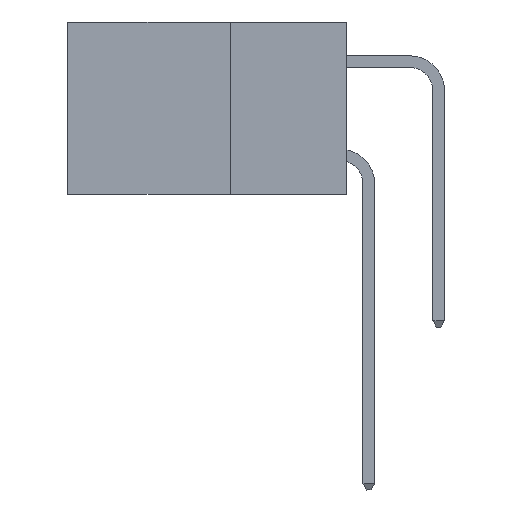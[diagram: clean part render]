
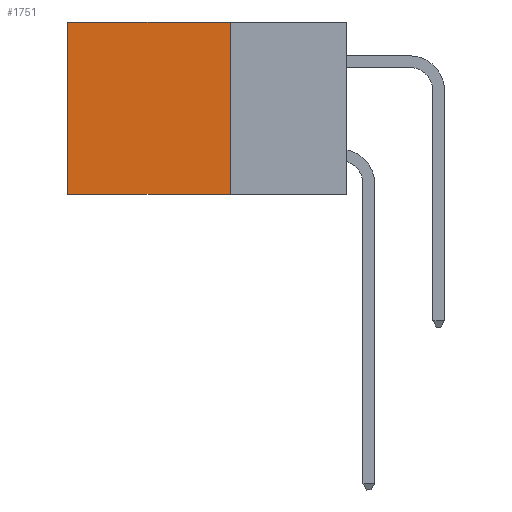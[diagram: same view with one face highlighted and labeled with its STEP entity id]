
A CAD part, left-side view. The second image highlights one B-rep face of the part: STEP entity #1751.
In plain terms, the highlighted planar face has unit normal (-1, 0, 0).
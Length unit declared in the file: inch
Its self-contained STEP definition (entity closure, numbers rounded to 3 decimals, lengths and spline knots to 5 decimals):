
#8 = DIRECTION ( 'NONE',  ( 0., 1., 0. ) ) ;
#408 = VERTEX_POINT ( 'NONE', #25837 ) ;
#820 = CARTESIAN_POINT ( 'NONE',  ( 0.2875, 0.25, -0.37 ) ) ;
#846 = VERTEX_POINT ( 'NONE', #19002 ) ;
#880 = FACE_OUTER_BOUND ( 'NONE', #23633, .T. ) ;
#1751 = ADVANCED_FACE ( 'NONE', ( #880 ), #26818, .F. ) ;
#1771 = VERTEX_POINT ( 'NONE', #12324 ) ;
#3113 = DIRECTION ( 'NONE',  ( 0., 0., -1. ) ) ;
#4030 = CARTESIAN_POINT ( 'NONE',  ( 0.2875, 0.25, 0. ) ) ;
#4594 = EDGE_CURVE ( 'NONE', #1771, #5830, #13624, .T. ) ;
#5017 = LINE ( 'NONE', #11598, #8546 ) ;
#5216 = VECTOR ( 'NONE', #19657, 39.37008 ) ;
#5830 = VERTEX_POINT ( 'NONE', #26468 ) ;
#8034 = CARTESIAN_POINT ( 'NONE',  ( 0.2875, 0.25, 0. ) ) ;
#8546 = VECTOR ( 'NONE', #11878, 39.37008 ) ;
#9437 = ORIENTED_EDGE ( 'NONE', *, *, #17806, .F. ) ;
#10472 = EDGE_CURVE ( 'NONE', #5830, #846, #19423, .T. ) ;
#11326 = CARTESIAN_POINT ( 'NONE',  ( 0.2875, 0.6, 0. ) ) ;
#11598 = CARTESIAN_POINT ( 'NONE',  ( 0.2875, 0.25, 0. ) ) ;
#11878 = DIRECTION ( 'NONE',  ( 0., 0., -1. ) ) ;
#12324 = CARTESIAN_POINT ( 'NONE',  ( 0.2875, 0.25, 0. ) ) ;
#13624 = LINE ( 'NONE', #8034, #25038 ) ;
#14179 = DIRECTION ( 'NONE',  ( 1., 0., 0. ) ) ;
#15277 = ORIENTED_EDGE ( 'NONE', *, *, #10472, .T. ) ;
#17806 = EDGE_CURVE ( 'NONE', #408, #846, #18508, .T. ) ;
#18508 = LINE ( 'NONE', #820, #5216 ) ;
#18568 = ORIENTED_EDGE ( 'NONE', *, *, #4594, .T. ) ;
#19002 = CARTESIAN_POINT ( 'NONE',  ( 0.2875, 0.6, -0.37 ) ) ;
#19423 = LINE ( 'NONE', #11326, #23628 ) ;
#19657 = DIRECTION ( 'NONE',  ( 0., 1., 0. ) ) ;
#20728 = EDGE_CURVE ( 'NONE', #1771, #408, #5017, .T. ) ;
#23628 = VECTOR ( 'NONE', #3113, 39.37008 ) ;
#23633 = EDGE_LOOP ( 'NONE', ( #15277, #9437, #25301, #18568 ) ) ;
#24120 = AXIS2_PLACEMENT_3D ( 'NONE', #4030, #14179, #26728 ) ;
#25038 = VECTOR ( 'NONE', #8, 39.37008 ) ;
#25301 = ORIENTED_EDGE ( 'NONE', *, *, #20728, .F. ) ;
#25837 = CARTESIAN_POINT ( 'NONE',  ( 0.2875, 0.25, -0.37 ) ) ;
#26468 = CARTESIAN_POINT ( 'NONE',  ( 0.2875, 0.6, 0. ) ) ;
#26728 = DIRECTION ( 'NONE',  ( 0., 0., -1. ) ) ;
#26818 = PLANE ( 'NONE',  #24120 ) ;
